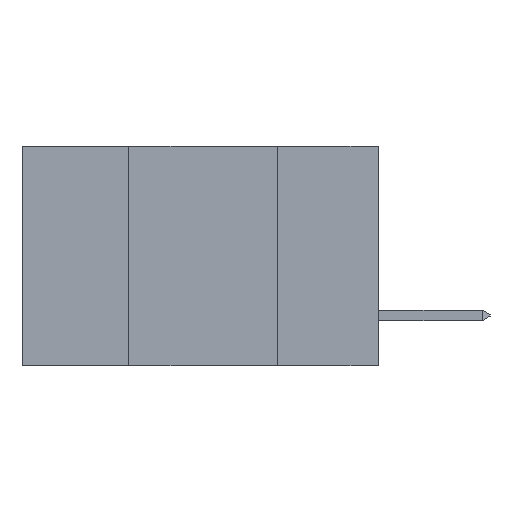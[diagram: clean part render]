
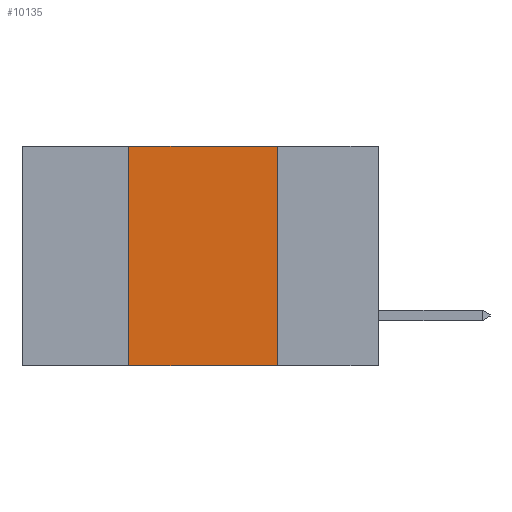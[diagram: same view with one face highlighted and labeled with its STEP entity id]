
A CAD part, left-side view. The second image highlights one B-rep face of the part: STEP entity #10135.
In plain terms, the highlighted planar face has unit normal (-1, 0, 0).
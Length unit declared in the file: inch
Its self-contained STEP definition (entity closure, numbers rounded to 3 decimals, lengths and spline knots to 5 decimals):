
#1014 = CARTESIAN_POINT ( 'NONE',  ( 0., 0.42, 0. ) ) ;
#1147 = CARTESIAN_POINT ( 'NONE',  ( 0., 0.42, -0.37 ) ) ;
#1237 = CARTESIAN_POINT ( 'NONE',  ( 0., 0.42, -0.37 ) ) ;
#1891 = EDGE_LOOP ( 'NONE', ( #12066, #4260, #5780, #17144 ) ) ;
#3244 = CARTESIAN_POINT ( 'NONE',  ( 0., 0.6, 0. ) ) ;
#3360 = EDGE_CURVE ( 'NONE', #7166, #16943, #7130, .T. ) ;
#3489 = VECTOR ( 'NONE', #10916, 39.37008 ) ;
#3648 = LINE ( 'NONE', #1147, #6864 ) ;
#4260 = ORIENTED_EDGE ( 'NONE', *, *, #13891, .F. ) ;
#5780 = ORIENTED_EDGE ( 'NONE', *, *, #12954, .F. ) ;
#5993 = PLANE ( 'NONE',  #16866 ) ;
#6122 = VERTEX_POINT ( 'NONE', #13558 ) ;
#6639 = VECTOR ( 'NONE', #10097, 39.37008 ) ;
#6864 = VECTOR ( 'NONE', #17536, 39.37008 ) ;
#7130 = LINE ( 'NONE', #11395, #3489 ) ;
#7166 = VERTEX_POINT ( 'NONE', #1237 ) ;
#7181 = VERTEX_POINT ( 'NONE', #1014 ) ;
#7371 = DIRECTION ( 'NONE',  ( 0., 0., -1. ) ) ;
#8701 = CARTESIAN_POINT ( 'NONE',  ( 0., 0.6, 0. ) ) ;
#9071 = VECTOR ( 'NONE', #13893, 39.37008 ) ;
#9265 = EDGE_CURVE ( 'NONE', #6122, #16943, #16334, .T. ) ;
#10097 = DIRECTION ( 'NONE',  ( 0., -1., 0. ) ) ;
#10135 = ADVANCED_FACE ( 'NONE', ( #17155 ), #5993, .F. ) ;
#10916 = DIRECTION ( 'NONE',  ( 0., -1., 0. ) ) ;
#11395 = CARTESIAN_POINT ( 'NONE',  ( 0., 0.6, -0.37 ) ) ;
#12066 = ORIENTED_EDGE ( 'NONE', *, *, #9265, .F. ) ;
#12489 = CARTESIAN_POINT ( 'NONE',  ( 0., 0.17, -0.37 ) ) ;
#12954 = EDGE_CURVE ( 'NONE', #7166, #7181, #3648, .T. ) ;
#13558 = CARTESIAN_POINT ( 'NONE',  ( 0., 0.17, 0. ) ) ;
#13891 = EDGE_CURVE ( 'NONE', #7181, #6122, #17159, .T. ) ;
#13893 = DIRECTION ( 'NONE',  ( 0., 0., -1. ) ) ;
#15639 = DIRECTION ( 'NONE',  ( 1., 0., 0. ) ) ;
#16129 = CARTESIAN_POINT ( 'NONE',  ( 0., 0.17, -0.37 ) ) ;
#16334 = LINE ( 'NONE', #12489, #9071 ) ;
#16866 = AXIS2_PLACEMENT_3D ( 'NONE', #3244, #15639, #7371 ) ;
#16943 = VERTEX_POINT ( 'NONE', #16129 ) ;
#17144 = ORIENTED_EDGE ( 'NONE', *, *, #3360, .T. ) ;
#17155 = FACE_OUTER_BOUND ( 'NONE', #1891, .T. ) ;
#17159 = LINE ( 'NONE', #8701, #6639 ) ;
#17536 = DIRECTION ( 'NONE',  ( 0., 0., 1. ) ) ;
